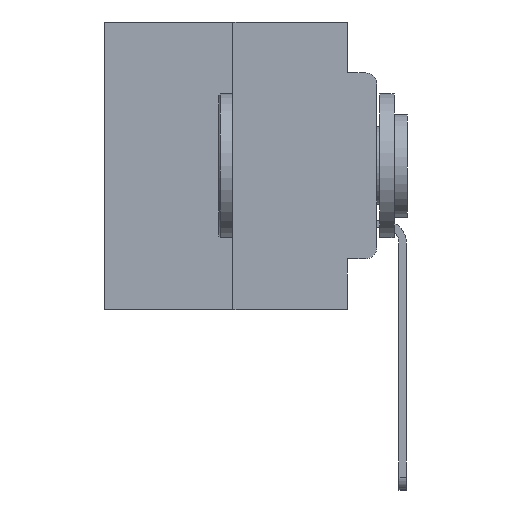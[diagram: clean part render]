
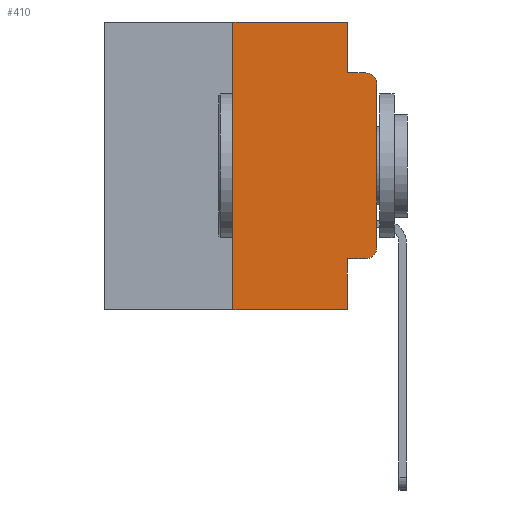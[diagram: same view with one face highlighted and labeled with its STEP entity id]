
A CAD part, left-side view. The second image highlights one B-rep face of the part: STEP entity #410.
In plain terms, the highlighted planar face has unit normal (-1, 0, 0).
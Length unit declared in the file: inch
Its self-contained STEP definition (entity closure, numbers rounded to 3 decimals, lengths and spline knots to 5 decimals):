
#81 = EDGE_CURVE ( 'NONE', #10998, #951, #5138, .T. ) ;
#91 = DIRECTION ( 'NONE',  ( 0., -1., 0. ) ) ;
#290 = CARTESIAN_POINT ( 'NONE',  ( 0., 0.473, 0. ) ) ;
#410 = ADVANCED_FACE ( 'NONE', ( #13743 ), #17775, .F. ) ;
#555 = LINE ( 'NONE', #24022, #11672 ) ;
#576 = EDGE_CURVE ( 'NONE', #3453, #26424, #20851, .T. ) ;
#951 = VERTEX_POINT ( 'NONE', #15087 ) ;
#1831 = DIRECTION ( 'NONE',  ( 0., 0., -1. ) ) ;
#1846 = LINE ( 'NONE', #290, #12884 ) ;
#1876 = VERTEX_POINT ( 'NONE', #10375 ) ;
#3059 = VECTOR ( 'NONE', #5885, 39.37008 ) ;
#3453 = VERTEX_POINT ( 'NONE', #8336 ) ;
#3480 = EDGE_CURVE ( 'NONE', #13056, #21661, #1846, .T. ) ;
#3501 = CARTESIAN_POINT ( 'NONE',  ( 0., 0.473, 0. ) ) ;
#3526 = EDGE_CURVE ( 'NONE', #1876, #951, #17830, .T. ) ;
#3649 = CARTESIAN_POINT ( 'NONE',  ( 0., 0.25, 0. ) ) ;
#4815 = ORIENTED_EDGE ( 'NONE', *, *, #3526, .T. ) ;
#5134 = ORIENTED_EDGE ( 'NONE', *, *, #3480, .F. ) ;
#5138 = LINE ( 'NONE', #10938, #26920 ) ;
#5143 = CARTESIAN_POINT ( 'NONE',  ( 0., 0.25, 0. ) ) ;
#5367 = AXIS2_PLACEMENT_3D ( 'NONE', #3501, #7531, #8309 ) ;
#5885 = DIRECTION ( 'NONE',  ( 0., 0., 1. ) ) ;
#6199 = LINE ( 'NONE', #21948, #17065 ) ;
#7531 = DIRECTION ( 'NONE',  ( 1., 0., 0. ) ) ;
#7654 = CIRCLE ( 'NONE', #20776, 0.02 ) ;
#8228 = DIRECTION ( 'NONE',  ( -1., 0., 0. ) ) ;
#8309 = DIRECTION ( 'NONE',  ( 0., 0., -1. ) ) ;
#8336 = CARTESIAN_POINT ( 'NONE',  ( 0., 0., -0.3915 ) ) ;
#10375 = CARTESIAN_POINT ( 'NONE',  ( 0., 0.25, -0.5 ) ) ;
#10938 = CARTESIAN_POINT ( 'NONE',  ( 0., 0.051, 0. ) ) ;
#10998 = VERTEX_POINT ( 'NONE', #25998 ) ;
#11456 = EDGE_CURVE ( 'NONE', #23677, #21492, #16154, .T. ) ;
#11672 = VECTOR ( 'NONE', #26101, 39.37008 ) ;
#12091 = CARTESIAN_POINT ( 'NONE',  ( 0., 0.02, -0.4115 ) ) ;
#12498 = EDGE_CURVE ( 'NONE', #21661, #23677, #6199, .T. ) ;
#12732 = ORIENTED_EDGE ( 'NONE', *, *, #81, .F. ) ;
#12884 = VECTOR ( 'NONE', #25871, 39.37008 ) ;
#12901 = CIRCLE ( 'NONE', #15424, 0.02 ) ;
#13056 = VERTEX_POINT ( 'NONE', #5143 ) ;
#13127 = VERTEX_POINT ( 'NONE', #12091 ) ;
#13506 = CARTESIAN_POINT ( 'NONE',  ( 0., 0.051, 0. ) ) ;
#13618 = CARTESIAN_POINT ( 'NONE',  ( 0., 0., -0.1085 ) ) ;
#13743 = FACE_OUTER_BOUND ( 'NONE', #23888, .T. ) ;
#14095 = ORIENTED_EDGE ( 'NONE', *, *, #11456, .F. ) ;
#14764 = LINE ( 'NONE', #3649, #3059 ) ;
#14984 = DIRECTION ( 'NONE',  ( -1., 0., 0. ) ) ;
#15087 = CARTESIAN_POINT ( 'NONE',  ( 0., 0.051, -0.5 ) ) ;
#15403 = ORIENTED_EDGE ( 'NONE', *, *, #12498, .F. ) ;
#15424 = AXIS2_PLACEMENT_3D ( 'NONE', #20959, #8228, #22984 ) ;
#16091 = ORIENTED_EDGE ( 'NONE', *, *, #26053, .T. ) ;
#16154 = LINE ( 'NONE', #19529, #26375 ) ;
#17065 = VECTOR ( 'NONE', #23996, 39.37008 ) ;
#17566 = CARTESIAN_POINT ( 'NONE',  ( 0., 0., 0. ) ) ;
#17775 = PLANE ( 'NONE',  #5367 ) ;
#17830 = LINE ( 'NONE', #24869, #22602 ) ;
#18309 = CARTESIAN_POINT ( 'NONE',  ( 0., 0.051, -0.0885 ) ) ;
#19208 = EDGE_CURVE ( 'NONE', #1876, #13056, #14764, .T. ) ;
#19529 = CARTESIAN_POINT ( 'NONE',  ( 0., 0.051, -0.0885 ) ) ;
#19561 = VECTOR ( 'NONE', #23654, 39.37008 ) ;
#19906 = ORIENTED_EDGE ( 'NONE', *, *, #19208, .F. ) ;
#20014 = EDGE_CURVE ( 'NONE', #10998, #13127, #555, .T. ) ;
#20247 = ORIENTED_EDGE ( 'NONE', *, *, #20014, .T. ) ;
#20776 = AXIS2_PLACEMENT_3D ( 'NONE', #27242, #14984, #1831 ) ;
#20851 = LINE ( 'NONE', #17566, #19561 ) ;
#20959 = CARTESIAN_POINT ( 'NONE',  ( 0., 0.02, -0.3915 ) ) ;
#21492 = VERTEX_POINT ( 'NONE', #26035 ) ;
#21587 = DIRECTION ( 'NONE',  ( 0., -1., 0. ) ) ;
#21661 = VERTEX_POINT ( 'NONE', #13506 ) ;
#21948 = CARTESIAN_POINT ( 'NONE',  ( 0., 0.051, 0. ) ) ;
#22602 = VECTOR ( 'NONE', #91, 39.37008 ) ;
#22984 = DIRECTION ( 'NONE',  ( 0., 0., -1. ) ) ;
#23073 = ORIENTED_EDGE ( 'NONE', *, *, #27522, .T. ) ;
#23654 = DIRECTION ( 'NONE',  ( 0., 0., 1. ) ) ;
#23677 = VERTEX_POINT ( 'NONE', #18309 ) ;
#23888 = EDGE_LOOP ( 'NONE', ( #26585, #23073, #14095, #15403, #5134, #19906, #4815, #12732, #20247, #16091 ) ) ;
#23996 = DIRECTION ( 'NONE',  ( 0., 0., -1. ) ) ;
#24022 = CARTESIAN_POINT ( 'NONE',  ( 0., 0.051, -0.4115 ) ) ;
#24869 = CARTESIAN_POINT ( 'NONE',  ( 0., 0.473, -0.5 ) ) ;
#25871 = DIRECTION ( 'NONE',  ( 0., -1., 0. ) ) ;
#25998 = CARTESIAN_POINT ( 'NONE',  ( 0., 0.051, -0.4115 ) ) ;
#26035 = CARTESIAN_POINT ( 'NONE',  ( 0., 0.02, -0.0885 ) ) ;
#26053 = EDGE_CURVE ( 'NONE', #13127, #3453, #12901, .T. ) ;
#26101 = DIRECTION ( 'NONE',  ( 0., -1., 0. ) ) ;
#26375 = VECTOR ( 'NONE', #21587, 39.37008 ) ;
#26424 = VERTEX_POINT ( 'NONE', #13618 ) ;
#26585 = ORIENTED_EDGE ( 'NONE', *, *, #576, .T. ) ;
#26920 = VECTOR ( 'NONE', #27168, 39.37008 ) ;
#27168 = DIRECTION ( 'NONE',  ( 0., 0., -1. ) ) ;
#27242 = CARTESIAN_POINT ( 'NONE',  ( 0., 0.02, -0.1085 ) ) ;
#27522 = EDGE_CURVE ( 'NONE', #26424, #21492, #7654, .T. ) ;
